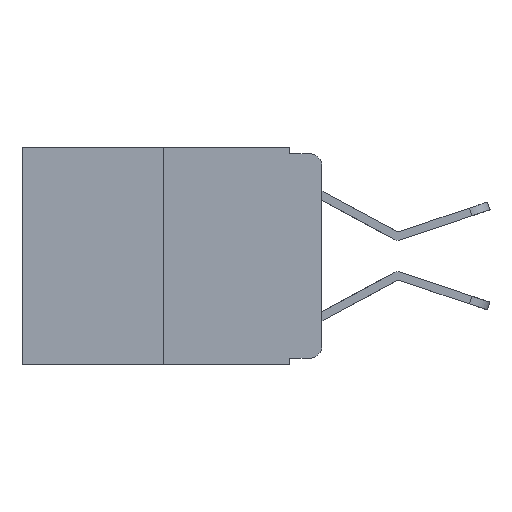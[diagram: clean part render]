
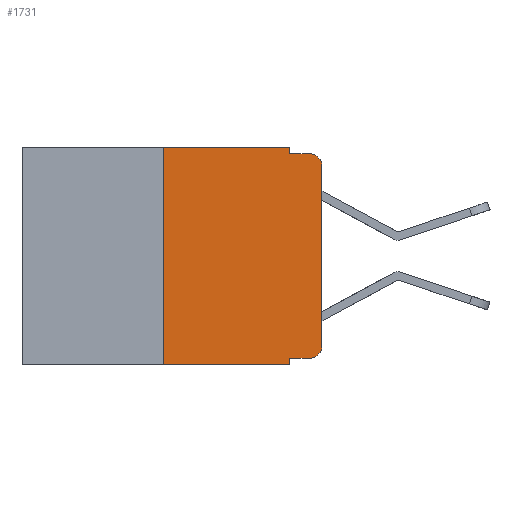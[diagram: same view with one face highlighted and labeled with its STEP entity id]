
A CAD part, left-side view. The second image highlights one B-rep face of the part: STEP entity #1731.
In plain terms, the highlighted planar face has unit normal (-1, 0, 0).
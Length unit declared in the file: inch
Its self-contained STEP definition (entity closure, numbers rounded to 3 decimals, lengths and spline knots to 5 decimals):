
#326 = VERTEX_POINT ( 'NONE', #466 ) ;
#466 = CARTESIAN_POINT ( 'NONE',  ( 0., 0., -0.313 ) ) ;
#476 = VECTOR ( 'NONE', #11149, 39.37008 ) ;
#518 = DIRECTION ( 'NONE',  ( 0., -1., 0. ) ) ;
#956 = CARTESIAN_POINT ( 'NONE',  ( 0., 0.051, 0. ) ) ;
#1389 = CARTESIAN_POINT ( 'NONE',  ( 0., 0.473, -0.343 ) ) ;
#1441 = CARTESIAN_POINT ( 'NONE',  ( 0., 0.051, 0. ) ) ;
#1460 = VECTOR ( 'NONE', #11073, 39.37008 ) ;
#1668 = DIRECTION ( 'NONE',  ( 0., -1., 0. ) ) ;
#1731 = ADVANCED_FACE ( 'NONE', ( #14469 ), #7618, .F. ) ;
#1932 = LINE ( 'NONE', #1389, #1460 ) ;
#2249 = CARTESIAN_POINT ( 'NONE',  ( 0., 0.02, -0.01 ) ) ;
#2888 = DIRECTION ( 'NONE',  ( 0., 0., -1. ) ) ;
#2893 = VERTEX_POINT ( 'NONE', #13143 ) ;
#3447 = CARTESIAN_POINT ( 'NONE',  ( 0., 0.051, -0.333 ) ) ;
#3970 = DIRECTION ( 'NONE',  ( -1., 0., 0. ) ) ;
#4048 = ORIENTED_EDGE ( 'NONE', *, *, #6402, .F. ) ;
#4056 = LINE ( 'NONE', #1441, #13698 ) ;
#4318 = LINE ( 'NONE', #5202, #476 ) ;
#4570 = EDGE_CURVE ( 'NONE', #5665, #10542, #14821, .T. ) ;
#4571 = ORIENTED_EDGE ( 'NONE', *, *, #4570, .F. ) ;
#5020 = CARTESIAN_POINT ( 'NONE',  ( 0., 0., -0.03 ) ) ;
#5029 = EDGE_CURVE ( 'NONE', #8907, #17479, #4318, .T. ) ;
#5135 = ORIENTED_EDGE ( 'NONE', *, *, #5029, .F. ) ;
#5202 = CARTESIAN_POINT ( 'NONE',  ( 0., 0.25, 0. ) ) ;
#5341 = DIRECTION ( 'NONE',  ( 0., 0., -1. ) ) ;
#5665 = VERTEX_POINT ( 'NONE', #15128 ) ;
#5913 = CARTESIAN_POINT ( 'NONE',  ( 0., 0.02, -0.03 ) ) ;
#5959 = EDGE_CURVE ( 'NONE', #5665, #2893, #9233, .T. ) ;
#6347 = AXIS2_PLACEMENT_3D ( 'NONE', #5913, #15454, #7302 ) ;
#6402 = EDGE_CURVE ( 'NONE', #12726, #14125, #4056, .T. ) ;
#6569 = CARTESIAN_POINT ( 'NONE',  ( 0., 0.051, 0. ) ) ;
#6679 = VECTOR ( 'NONE', #8762, 39.37008 ) ;
#7042 = LINE ( 'NONE', #9977, #10679 ) ;
#7122 = LINE ( 'NONE', #14209, #6679 ) ;
#7136 = CIRCLE ( 'NONE', #10997, 0.02 ) ;
#7302 = DIRECTION ( 'NONE',  ( 0., 0., -1. ) ) ;
#7345 = EDGE_LOOP ( 'NONE', ( #14182, #16727, #15869, #4048, #16671, #5135, #16532, #4571, #13922, #11747 ) ) ;
#7456 = CARTESIAN_POINT ( 'NONE',  ( 0., 0.051, -0.343 ) ) ;
#7618 = PLANE ( 'NONE',  #8324 ) ;
#8187 = EDGE_CURVE ( 'NONE', #8413, #10120, #12547, .T. ) ;
#8324 = AXIS2_PLACEMENT_3D ( 'NONE', #10872, #13376, #9122 ) ;
#8350 = DIRECTION ( 'NONE',  ( 0., -1., 0. ) ) ;
#8413 = VERTEX_POINT ( 'NONE', #5020 ) ;
#8662 = EDGE_CURVE ( 'NONE', #14125, #10120, #16155, .T. ) ;
#8762 = DIRECTION ( 'NONE',  ( 0., 0., 1. ) ) ;
#8879 = CARTESIAN_POINT ( 'NONE',  ( 0., 0.25, -0.343 ) ) ;
#8907 = VERTEX_POINT ( 'NONE', #8879 ) ;
#9122 = DIRECTION ( 'NONE',  ( 0., 0., -1. ) ) ;
#9233 = LINE ( 'NONE', #3447, #16050 ) ;
#9286 = EDGE_CURVE ( 'NONE', #8907, #10542, #1932, .T. ) ;
#9977 = CARTESIAN_POINT ( 'NONE',  ( 0., 0.473, 0. ) ) ;
#10120 = VERTEX_POINT ( 'NONE', #2249 ) ;
#10490 = EDGE_CURVE ( 'NONE', #326, #8413, #7122, .T. ) ;
#10542 = VERTEX_POINT ( 'NONE', #7456 ) ;
#10679 = VECTOR ( 'NONE', #1668, 39.37008 ) ;
#10872 = CARTESIAN_POINT ( 'NONE',  ( 0., 0.473, 0. ) ) ;
#10997 = AXIS2_PLACEMENT_3D ( 'NONE', #12210, #3970, #13572 ) ;
#11033 = CARTESIAN_POINT ( 'NONE',  ( 0., 0.051, -0.01 ) ) ;
#11073 = DIRECTION ( 'NONE',  ( 0., -1., 0. ) ) ;
#11149 = DIRECTION ( 'NONE',  ( 0., 0., 1. ) ) ;
#11200 = VECTOR ( 'NONE', #5341, 39.37008 ) ;
#11747 = ORIENTED_EDGE ( 'NONE', *, *, #14668, .T. ) ;
#12210 = CARTESIAN_POINT ( 'NONE',  ( 0., 0.02, -0.313 ) ) ;
#12362 = EDGE_CURVE ( 'NONE', #17479, #12726, #7042, .T. ) ;
#12547 = CIRCLE ( 'NONE', #6347, 0.02 ) ;
#12726 = VERTEX_POINT ( 'NONE', #956 ) ;
#13143 = CARTESIAN_POINT ( 'NONE',  ( 0., 0.02, -0.333 ) ) ;
#13376 = DIRECTION ( 'NONE',  ( 1., 0., 0. ) ) ;
#13572 = DIRECTION ( 'NONE',  ( 0., 0., -1. ) ) ;
#13698 = VECTOR ( 'NONE', #2888, 39.37008 ) ;
#13922 = ORIENTED_EDGE ( 'NONE', *, *, #5959, .T. ) ;
#14125 = VERTEX_POINT ( 'NONE', #15227 ) ;
#14182 = ORIENTED_EDGE ( 'NONE', *, *, #10490, .T. ) ;
#14209 = CARTESIAN_POINT ( 'NONE',  ( 0., 0., 0. ) ) ;
#14467 = VECTOR ( 'NONE', #8350, 39.37008 ) ;
#14469 = FACE_OUTER_BOUND ( 'NONE', #7345, .T. ) ;
#14668 = EDGE_CURVE ( 'NONE', #2893, #326, #7136, .T. ) ;
#14821 = LINE ( 'NONE', #6569, #11200 ) ;
#15128 = CARTESIAN_POINT ( 'NONE',  ( 0., 0.051, -0.333 ) ) ;
#15227 = CARTESIAN_POINT ( 'NONE',  ( 0., 0.051, -0.01 ) ) ;
#15454 = DIRECTION ( 'NONE',  ( -1., 0., 0. ) ) ;
#15869 = ORIENTED_EDGE ( 'NONE', *, *, #8662, .F. ) ;
#16050 = VECTOR ( 'NONE', #518, 39.37008 ) ;
#16155 = LINE ( 'NONE', #11033, #14467 ) ;
#16532 = ORIENTED_EDGE ( 'NONE', *, *, #9286, .T. ) ;
#16671 = ORIENTED_EDGE ( 'NONE', *, *, #12362, .F. ) ;
#16727 = ORIENTED_EDGE ( 'NONE', *, *, #8187, .T. ) ;
#17228 = CARTESIAN_POINT ( 'NONE',  ( 0., 0.25, 0. ) ) ;
#17479 = VERTEX_POINT ( 'NONE', #17228 ) ;
